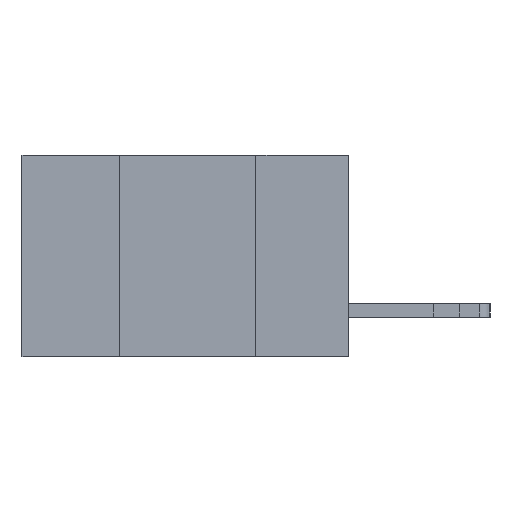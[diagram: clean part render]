
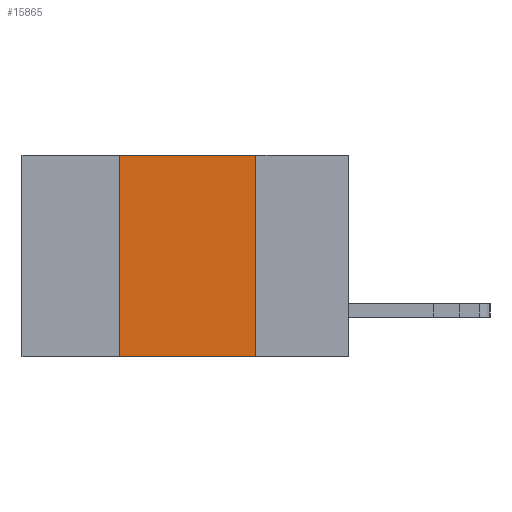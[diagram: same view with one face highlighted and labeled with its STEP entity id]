
A CAD part, left-side view. The second image highlights one B-rep face of the part: STEP entity #15865.
In plain terms, the highlighted planar face has unit normal (-1, 0, 0).
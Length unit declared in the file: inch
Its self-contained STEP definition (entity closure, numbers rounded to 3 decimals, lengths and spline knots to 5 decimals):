
#356 = DIRECTION ( 'NONE',  ( 0., 0., -1. ) ) ;
#805 = LINE ( 'NONE', #22148, #24778 ) ;
#1264 = LINE ( 'NONE', #19613, #16850 ) ;
#1521 = DIRECTION ( 'NONE',  ( 0., -1., 0. ) ) ;
#1943 = VERTEX_POINT ( 'NONE', #19392 ) ;
#1974 = CARTESIAN_POINT ( 'NONE',  ( 0., 0.6, 0. ) ) ;
#2199 = DIRECTION ( 'NONE',  ( 0., 0., -1. ) ) ;
#5218 = EDGE_CURVE ( 'NONE', #14145, #1943, #805, .T. ) ;
#6978 = ORIENTED_EDGE ( 'NONE', *, *, #7690, .F. ) ;
#7606 = ORIENTED_EDGE ( 'NONE', *, *, #5218, .T. ) ;
#7690 = EDGE_CURVE ( 'NONE', #14145, #8932, #1264, .T. ) ;
#7838 = LINE ( 'NONE', #17732, #11867 ) ;
#8445 = CARTESIAN_POINT ( 'NONE',  ( 0., 0.42, 0. ) ) ;
#8932 = VERTEX_POINT ( 'NONE', #8445 ) ;
#10258 = FACE_OUTER_BOUND ( 'NONE', #16756, .T. ) ;
#11126 = VERTEX_POINT ( 'NONE', #21877 ) ;
#11867 = VECTOR ( 'NONE', #2199, 39.37008 ) ;
#12060 = DIRECTION ( 'NONE',  ( 1., 0., 0. ) ) ;
#13365 = EDGE_CURVE ( 'NONE', #8932, #11126, #18571, .T. ) ;
#13770 = ORIENTED_EDGE ( 'NONE', *, *, #14118, .F. ) ;
#14118 = EDGE_CURVE ( 'NONE', #11126, #1943, #7838, .T. ) ;
#14145 = VERTEX_POINT ( 'NONE', #15852 ) ;
#15852 = CARTESIAN_POINT ( 'NONE',  ( 0., 0.42, -0.37 ) ) ;
#15865 = ADVANCED_FACE ( 'NONE', ( #10258 ), #19821, .F. ) ;
#16756 = EDGE_LOOP ( 'NONE', ( #13770, #19540, #6978, #7606 ) ) ;
#16850 = VECTOR ( 'NONE', #19869, 39.37008 ) ;
#17590 = DIRECTION ( 'NONE',  ( 0., -1., 0. ) ) ;
#17732 = CARTESIAN_POINT ( 'NONE',  ( 0., 0.17, 0. ) ) ;
#18571 = LINE ( 'NONE', #1974, #19178 ) ;
#19178 = VECTOR ( 'NONE', #17590, 39.37008 ) ;
#19392 = CARTESIAN_POINT ( 'NONE',  ( 0., 0.17, -0.37 ) ) ;
#19540 = ORIENTED_EDGE ( 'NONE', *, *, #13365, .F. ) ;
#19613 = CARTESIAN_POINT ( 'NONE',  ( 0., 0.42, 0. ) ) ;
#19700 = AXIS2_PLACEMENT_3D ( 'NONE', #23635, #12060, #356 ) ;
#19821 = PLANE ( 'NONE',  #19700 ) ;
#19869 = DIRECTION ( 'NONE',  ( 0., 0., 1. ) ) ;
#21877 = CARTESIAN_POINT ( 'NONE',  ( 0., 0.17, 0. ) ) ;
#22148 = CARTESIAN_POINT ( 'NONE',  ( 0., 0.6, -0.37 ) ) ;
#23635 = CARTESIAN_POINT ( 'NONE',  ( 0., 0.6, 0. ) ) ;
#24778 = VECTOR ( 'NONE', #1521, 39.37008 ) ;
